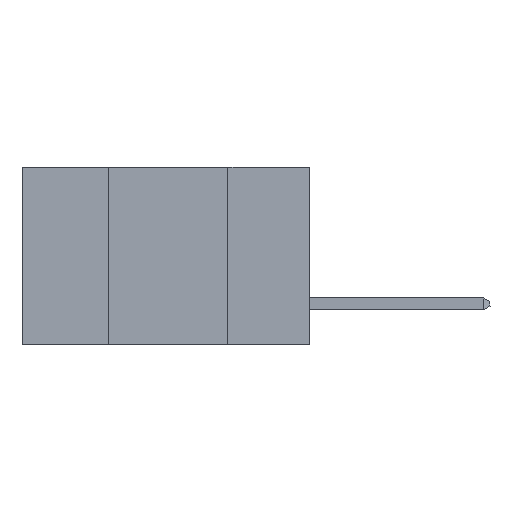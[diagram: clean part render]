
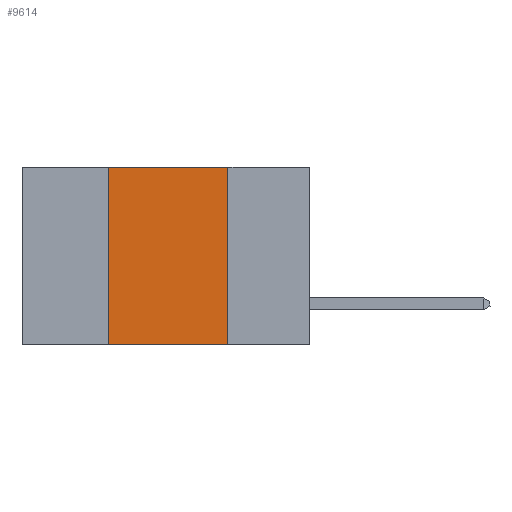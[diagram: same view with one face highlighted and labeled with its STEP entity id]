
A CAD part, left-side view. The second image highlights one B-rep face of the part: STEP entity #9614.
In plain terms, the highlighted planar face has unit normal (-1, 0, 0).
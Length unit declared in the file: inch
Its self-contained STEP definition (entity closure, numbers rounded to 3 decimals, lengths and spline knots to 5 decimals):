
#158 = VERTEX_POINT ( 'NONE', #31364 ) ;
#682 = DIRECTION ( 'NONE',  ( 0., 0., -1. ) ) ;
#1139 = ORIENTED_EDGE ( 'NONE', *, *, #6676, .F. ) ;
#1255 = EDGE_CURVE ( 'NONE', #11147, #28214, #30231, .T. ) ;
#1658 = EDGE_CURVE ( 'NONE', #11147, #158, #24112, .T. ) ;
#3473 = VECTOR ( 'NONE', #32543, 39.37008 ) ;
#3541 = CARTESIAN_POINT ( 'NONE',  ( 0., 0.17, 0. ) ) ;
#4134 = CARTESIAN_POINT ( 'NONE',  ( 0., 0.42, 0. ) ) ;
#5222 = ORIENTED_EDGE ( 'NONE', *, *, #1255, .T. ) ;
#6676 = EDGE_CURVE ( 'NONE', #158, #7958, #28524, .T. ) ;
#7544 = VECTOR ( 'NONE', #13338, 39.37008 ) ;
#7958 = VERTEX_POINT ( 'NONE', #25405 ) ;
#9614 = ADVANCED_FACE ( 'NONE', ( #24692 ), #27014, .F. ) ;
#10560 = LINE ( 'NONE', #3541, #3473 ) ;
#10677 = CARTESIAN_POINT ( 'NONE',  ( 0., 0.6, 0. ) ) ;
#10733 = ORIENTED_EDGE ( 'NONE', *, *, #27453, .F. ) ;
#11115 = EDGE_LOOP ( 'NONE', ( #10733, #1139, #15243, #5222 ) ) ;
#11147 = VERTEX_POINT ( 'NONE', #14713 ) ;
#13338 = DIRECTION ( 'NONE',  ( 0., -1., 0. ) ) ;
#14713 = CARTESIAN_POINT ( 'NONE',  ( 0., 0.42, -0.37 ) ) ;
#15243 = ORIENTED_EDGE ( 'NONE', *, *, #1658, .F. ) ;
#16305 = VECTOR ( 'NONE', #28924, 39.37008 ) ;
#16562 = DIRECTION ( 'NONE',  ( 1., 0., 0. ) ) ;
#17086 = VECTOR ( 'NONE', #20076, 39.37008 ) ;
#20076 = DIRECTION ( 'NONE',  ( 0., 0., 1. ) ) ;
#24112 = LINE ( 'NONE', #4134, #17086 ) ;
#24692 = FACE_OUTER_BOUND ( 'NONE', #11115, .T. ) ;
#25405 = CARTESIAN_POINT ( 'NONE',  ( 0., 0.17, 0. ) ) ;
#26300 = CARTESIAN_POINT ( 'NONE',  ( 0., 0.6, -0.37 ) ) ;
#27014 = PLANE ( 'NONE',  #32167 ) ;
#27453 = EDGE_CURVE ( 'NONE', #7958, #28214, #10560, .T. ) ;
#28214 = VERTEX_POINT ( 'NONE', #31494 ) ;
#28524 = LINE ( 'NONE', #10677, #7544 ) ;
#28924 = DIRECTION ( 'NONE',  ( 0., -1., 0. ) ) ;
#30231 = LINE ( 'NONE', #26300, #16305 ) ;
#31364 = CARTESIAN_POINT ( 'NONE',  ( 0., 0.42, 0. ) ) ;
#31494 = CARTESIAN_POINT ( 'NONE',  ( 0., 0.17, -0.37 ) ) ;
#32167 = AXIS2_PLACEMENT_3D ( 'NONE', #32251, #16562, #682 ) ;
#32251 = CARTESIAN_POINT ( 'NONE',  ( 0., 0.6, 0. ) ) ;
#32543 = DIRECTION ( 'NONE',  ( 0., 0., -1. ) ) ;
